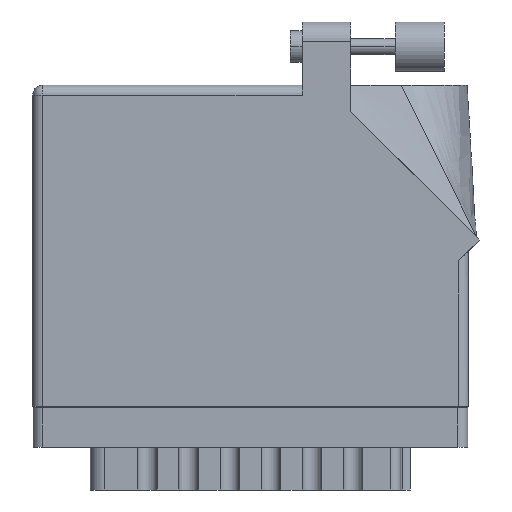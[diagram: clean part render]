
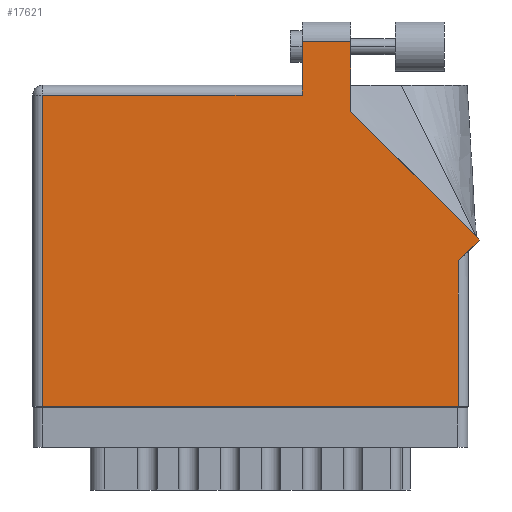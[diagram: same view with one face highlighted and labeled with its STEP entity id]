
A CAD part, front view. The second image highlights one B-rep face of the part: STEP entity #17621.
In plain terms, the highlighted face is planar.
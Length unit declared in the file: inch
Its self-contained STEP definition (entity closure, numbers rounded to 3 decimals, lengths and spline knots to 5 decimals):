
#651 = DIRECTION ( 'NONE',  ( 0., 1., 0. ) ) ;
#688 = ORIENTED_EDGE ( 'NONE', *, *, #54461, .T. ) ;
#3589 = EDGE_CURVE ( 'NONE', #19243, #10015, #80714, .T. ) ;
#5984 = VERTEX_POINT ( 'NONE', #75313 ) ;
#6677 = VECTOR ( 'NONE', #7894, 39.37008 ) ;
#7894 = DIRECTION ( 'NONE',  ( -1., 0., 0. ) ) ;
#7950 = VECTOR ( 'NONE', #68854, 39.37008 ) ;
#9142 = CARTESIAN_POINT ( 'NONE',  ( 0., 0., 0. ) ) ;
#10015 = VERTEX_POINT ( 'NONE', #50053 ) ;
#11283 = VECTOR ( 'NONE', #74356, 39.37008 ) ;
#11743 = PLANE ( 'NONE',  #80772 ) ;
#14235 = VECTOR ( 'NONE', #47872, 39.37008 ) ;
#16226 = CARTESIAN_POINT ( 'NONE',  ( 1.705, 2.03, 0. ) ) ;
#17621 = ADVANCED_FACE ( 'NONE', ( #22899 ), #11743, .F. ) ;
#19243 = VERTEX_POINT ( 'NONE', #76482 ) ;
#20493 = CARTESIAN_POINT ( 'NONE',  ( 2.012, 1.86442, 0. ) ) ;
#21004 = CARTESIAN_POINT ( 'NONE',  ( 1.705, 2.305, 0. ) ) ;
#21652 = EDGE_CURVE ( 'NONE', #10015, #35301, #85197, .T. ) ;
#22781 = CARTESIAN_POINT ( 'NONE',  ( 2.82571, 1.05071, 0. ) ) ;
#22899 = FACE_OUTER_BOUND ( 'NONE', #53598, .T. ) ;
#26719 = VERTEX_POINT ( 'NONE', #71647 ) ;
#27223 = ORIENTED_EDGE ( 'NONE', *, *, #33405, .T. ) ;
#28172 = ORIENTED_EDGE ( 'NONE', *, *, #57118, .T. ) ;
#28951 = EDGE_CURVE ( 'NONE', #65833, #84742, #79315, .T. ) ;
#29059 = LINE ( 'NONE', #21004, #11283 ) ;
#29917 = CARTESIAN_POINT ( 'NONE',  ( 2.755, 0.98, 0. ) ) ;
#33405 = EDGE_CURVE ( 'NONE', #35301, #26719, #84614, .T. ) ;
#34491 = VECTOR ( 'NONE', #43561, 39.37008 ) ;
#34650 = ORIENTED_EDGE ( 'NONE', *, *, #28951, .T. ) ;
#34971 = EDGE_CURVE ( 'NONE', #5984, #77236, #76989, .T. ) ;
#35301 = VERTEX_POINT ( 'NONE', #79333 ) ;
#35831 = DIRECTION ( 'NONE',  ( 0., -1., 0. ) ) ;
#35954 = DIRECTION ( 'NONE',  ( 0., 1., 0. ) ) ;
#37524 = CARTESIAN_POINT ( 'NONE',  ( 2.012, 2.305, 0. ) ) ;
#38869 = DIRECTION ( 'NONE',  ( -1., 0., 0. ) ) ;
#42118 = CARTESIAN_POINT ( 'NONE',  ( 2.82571, 1.05071, 0. ) ) ;
#43561 = DIRECTION ( 'NONE',  ( 0.707, 0.707, 0. ) ) ;
#44562 = ORIENTED_EDGE ( 'NONE', *, *, #3589, .T. ) ;
#47574 = ORIENTED_EDGE ( 'NONE', *, *, #58664, .T. ) ;
#47872 = DIRECTION ( 'NONE',  ( 0., -1., 0. ) ) ;
#50053 = CARTESIAN_POINT ( 'NONE',  ( 0.062, 1.968, 0. ) ) ;
#53598 = EDGE_LOOP ( 'NONE', ( #53888, #54924, #688, #44562, #55478, #27223, #47574, #34650, #28172 ) ) ;
#53888 = ORIENTED_EDGE ( 'NONE', *, *, #34971, .T. ) ;
#54461 = EDGE_CURVE ( 'NONE', #80280, #19243, #77179, .T. ) ;
#54924 = ORIENTED_EDGE ( 'NONE', *, *, #74643, .T. ) ;
#55478 = ORIENTED_EDGE ( 'NONE', *, *, #21652, .T. ) ;
#57118 = EDGE_CURVE ( 'NONE', #84742, #5984, #70520, .T. ) ;
#58397 = VECTOR ( 'NONE', #35831, 39.37008 ) ;
#58423 = DIRECTION ( 'NONE',  ( 0., 0., -1. ) ) ;
#58664 = EDGE_CURVE ( 'NONE', #26719, #65833, #81279, .T. ) ;
#59617 = VECTOR ( 'NONE', #68613, 39.37008 ) ;
#61029 = CARTESIAN_POINT ( 'NONE',  ( 1.705, 2.305, 0. ) ) ;
#65186 = CARTESIAN_POINT ( 'NONE',  ( 0.062, 0., 0. ) ) ;
#65702 = CARTESIAN_POINT ( 'NONE',  ( 0., 2.03, 0. ) ) ;
#65833 = VERTEX_POINT ( 'NONE', #80414 ) ;
#65935 = CARTESIAN_POINT ( 'NONE',  ( 0., 1.968, 0. ) ) ;
#68613 = DIRECTION ( 'NONE',  ( 1., 0., 0. ) ) ;
#68854 = DIRECTION ( 'NONE',  ( -0.707, 0.707, 0. ) ) ;
#70520 = LINE ( 'NONE', #22781, #7950 ) ;
#71647 = CARTESIAN_POINT ( 'NONE',  ( 2.693, 0., 0. ) ) ;
#74356 = DIRECTION ( 'NONE',  ( -1., 0., 0. ) ) ;
#74643 = EDGE_CURVE ( 'NONE', #77236, #80280, #29059, .T. ) ;
#75313 = CARTESIAN_POINT ( 'NONE',  ( 2.012, 1.86442, 0. ) ) ;
#75862 = CARTESIAN_POINT ( 'NONE',  ( 2.693, 0.98, 0. ) ) ;
#76482 = CARTESIAN_POINT ( 'NONE',  ( 1.705, 1.968, 0. ) ) ;
#76989 = LINE ( 'NONE', #20493, #81178 ) ;
#77179 = LINE ( 'NONE', #16226, #58397 ) ;
#77236 = VERTEX_POINT ( 'NONE', #37524 ) ;
#79315 = LINE ( 'NONE', #29917, #34491 ) ;
#79333 = CARTESIAN_POINT ( 'NONE',  ( 0.062, 0., 0. ) ) ;
#80280 = VERTEX_POINT ( 'NONE', #61029 ) ;
#80414 = CARTESIAN_POINT ( 'NONE',  ( 2.693, 0.918, 0. ) ) ;
#80714 = LINE ( 'NONE', #65935, #6677 ) ;
#80772 = AXIS2_PLACEMENT_3D ( 'NONE', #65702, #58423, #38869 ) ;
#81178 = VECTOR ( 'NONE', #651, 39.37008 ) ;
#81279 = LINE ( 'NONE', #75862, #83379 ) ;
#83379 = VECTOR ( 'NONE', #35954, 39.37008 ) ;
#84614 = LINE ( 'NONE', #9142, #59617 ) ;
#84742 = VERTEX_POINT ( 'NONE', #42118 ) ;
#85197 = LINE ( 'NONE', #65186, #14235 ) ;
